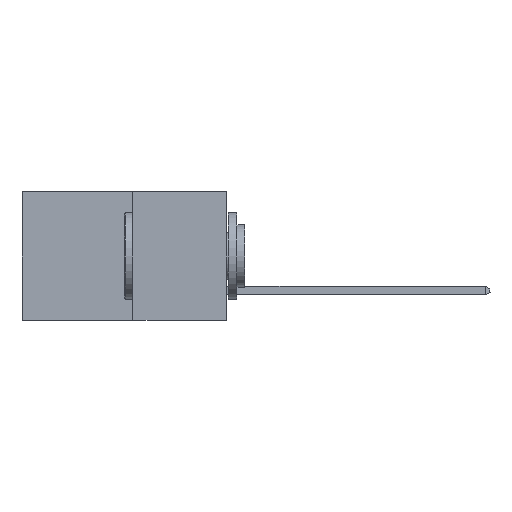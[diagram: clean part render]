
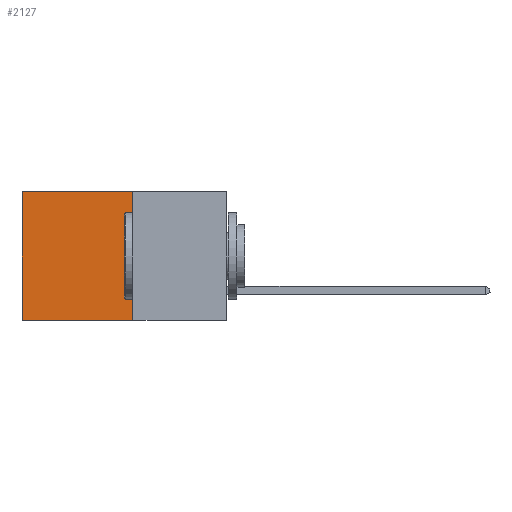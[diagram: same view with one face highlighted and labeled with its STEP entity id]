
A CAD part, left-side view. The second image highlights one B-rep face of the part: STEP entity #2127.
In plain terms, the highlighted planar face has unit normal (-1, 0, 0).
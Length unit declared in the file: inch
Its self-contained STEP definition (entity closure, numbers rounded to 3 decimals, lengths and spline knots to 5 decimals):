
#217 = CARTESIAN_POINT ( 'NONE',  ( 0.277, 0.27, -0.37 ) ) ;
#412 = ORIENTED_EDGE ( 'NONE', *, *, #13217, .F. ) ;
#760 = DIRECTION ( 'NONE',  ( 0., 1., 0. ) ) ;
#1551 = CARTESIAN_POINT ( 'NONE',  ( 0.277, 0.59, -0.37 ) ) ;
#1842 = CARTESIAN_POINT ( 'NONE',  ( 0.277, 0.27, 0. ) ) ;
#2127 = ADVANCED_FACE ( 'NONE', ( #2619 ), #6091, .F. ) ;
#2257 = EDGE_CURVE ( 'NONE', #5658, #8113, #12587, .T. ) ;
#2619 = FACE_OUTER_BOUND ( 'NONE', #8716, .T. ) ;
#3550 = EDGE_CURVE ( 'NONE', #9863, #5658, #5279, .T. ) ;
#3564 = CARTESIAN_POINT ( 'NONE',  ( 0.277, 0.27, 0. ) ) ;
#3582 = DIRECTION ( 'NONE',  ( 0., 1., 0. ) ) ;
#4708 = VECTOR ( 'NONE', #760, 39.37008 ) ;
#4717 = DIRECTION ( 'NONE',  ( 0., 0., -1. ) ) ;
#4730 = DIRECTION ( 'NONE',  ( 1., 0., 0. ) ) ;
#4798 = CARTESIAN_POINT ( 'NONE',  ( 0.277, 0.59, 0. ) ) ;
#4945 = CARTESIAN_POINT ( 'NONE',  ( 0.277, 0.27, -0.37 ) ) ;
#5279 = LINE ( 'NONE', #3564, #5952 ) ;
#5658 = VERTEX_POINT ( 'NONE', #4798 ) ;
#5736 = ORIENTED_EDGE ( 'NONE', *, *, #2257, .T. ) ;
#5952 = VECTOR ( 'NONE', #3582, 39.37008 ) ;
#6091 = PLANE ( 'NONE',  #8552 ) ;
#6449 = EDGE_CURVE ( 'NONE', #8824, #8113, #7479, .T. ) ;
#6778 = CARTESIAN_POINT ( 'NONE',  ( 0.277, 0.59, -0.37 ) ) ;
#7006 = CARTESIAN_POINT ( 'NONE',  ( 0.277, 0.27, -0.37 ) ) ;
#7479 = LINE ( 'NONE', #12222, #4708 ) ;
#7770 = DIRECTION ( 'NONE',  ( 0., 0., -1. ) ) ;
#8113 = VERTEX_POINT ( 'NONE', #1551 ) ;
#8492 = ORIENTED_EDGE ( 'NONE', *, *, #6449, .F. ) ;
#8552 = AXIS2_PLACEMENT_3D ( 'NONE', #7006, #4730, #4717 ) ;
#8716 = EDGE_LOOP ( 'NONE', ( #5736, #8492, #412, #8825 ) ) ;
#8789 = LINE ( 'NONE', #4945, #10873 ) ;
#8824 = VERTEX_POINT ( 'NONE', #217 ) ;
#8825 = ORIENTED_EDGE ( 'NONE', *, *, #3550, .T. ) ;
#9863 = VERTEX_POINT ( 'NONE', #1842 ) ;
#9869 = VECTOR ( 'NONE', #7770, 39.37008 ) ;
#10873 = VECTOR ( 'NONE', #11147, 39.37008 ) ;
#11147 = DIRECTION ( 'NONE',  ( 0., 0., -1. ) ) ;
#12222 = CARTESIAN_POINT ( 'NONE',  ( 0.277, 0.27, -0.37 ) ) ;
#12587 = LINE ( 'NONE', #6778, #9869 ) ;
#13217 = EDGE_CURVE ( 'NONE', #9863, #8824, #8789, .T. ) ;
